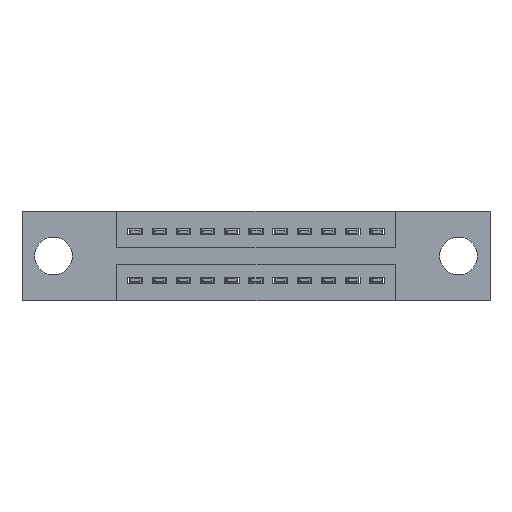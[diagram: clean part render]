
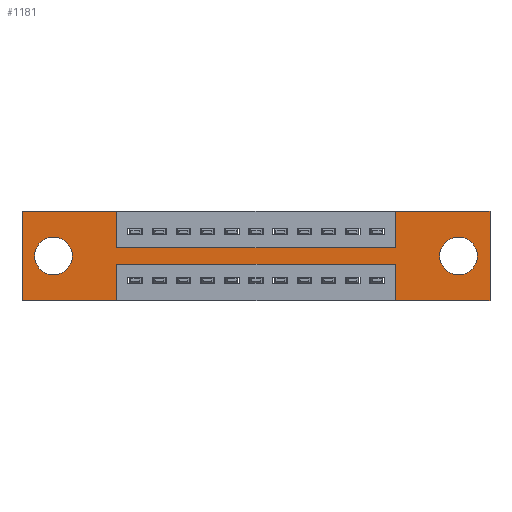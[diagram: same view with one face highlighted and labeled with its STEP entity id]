
A CAD part, front view. The second image highlights one B-rep face of the part: STEP entity #1181.
In plain terms, the highlighted planar face has unit normal (0, -1, 0).
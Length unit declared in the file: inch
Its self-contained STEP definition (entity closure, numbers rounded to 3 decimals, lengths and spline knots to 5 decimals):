
#24 = DIRECTION ( 'NONE',  ( 0., 0., -1. ) ) ;
#165 = EDGE_CURVE ( 'NONE', #11801, #4384, #6008, .T. ) ;
#247 = ORIENTED_EDGE ( 'NONE', *, *, #9492, .T. ) ;
#303 = DIRECTION ( 'NONE',  ( 0., 1., 0. ) ) ;
#377 = LINE ( 'NONE', #9774, #10524 ) ;
#446 = LINE ( 'NONE', #3167, #5166 ) ;
#485 = VECTOR ( 'NONE', #6870, 39.37008 ) ;
#511 = AXIS2_PLACEMENT_3D ( 'NONE', #3338, #11051, #2813 ) ;
#535 = CARTESIAN_POINT ( 'NONE',  ( 0.3925, 0., -0.15 ) ) ;
#619 = VECTOR ( 'NONE', #7497, 39.37008 ) ;
#682 = LINE ( 'NONE', #7815, #6014 ) ;
#769 = CIRCLE ( 'NONE', #1543, 0.078 ) ;
#784 = LINE ( 'NONE', #3765, #8325 ) ;
#936 = VECTOR ( 'NONE', #9405, 39.37008 ) ;
#1005 = VERTEX_POINT ( 'NONE', #3651 ) ;
#1015 = VERTEX_POINT ( 'NONE', #7721 ) ;
#1137 = ORIENTED_EDGE ( 'NONE', *, *, #5476, .F. ) ;
#1178 = CARTESIAN_POINT ( 'NONE',  ( 0.3925, 0., -0.22 ) ) ;
#1181 = ADVANCED_FACE ( 'NONE', ( #12139, #7328, #7035 ), #2074, .T. ) ;
#1235 = CARTESIAN_POINT ( 'NONE',  ( 1.805, 0., -0.185 ) ) ;
#1338 = DIRECTION ( 'NONE',  ( 0., 1., 0. ) ) ;
#1355 = EDGE_CURVE ( 'NONE', #3964, #2586, #2855, .T. ) ;
#1472 = ORIENTED_EDGE ( 'NONE', *, *, #9036, .F. ) ;
#1543 = AXIS2_PLACEMENT_3D ( 'NONE', #1235, #303, #24 ) ;
#1653 = VERTEX_POINT ( 'NONE', #2843 ) ;
#1767 = EDGE_CURVE ( 'NONE', #6382, #9145, #5819, .T. ) ;
#1768 = DIRECTION ( 'NONE',  ( 0., 0., -1. ) ) ;
#1961 = DIRECTION ( 'NONE',  ( 0., 0., -1. ) ) ;
#1983 = LINE ( 'NONE', #10677, #4322 ) ;
#2074 = PLANE ( 'NONE',  #511 ) ;
#2124 = CARTESIAN_POINT ( 'NONE',  ( 0.13, 0., -0.263 ) ) ;
#2142 = EDGE_CURVE ( 'NONE', #12505, #1005, #784, .T. ) ;
#2246 = CARTESIAN_POINT ( 'NONE',  ( 0., 0., 0. ) ) ;
#2266 = DIRECTION ( 'NONE',  ( -1., 0., 0. ) ) ;
#2586 = VERTEX_POINT ( 'NONE', #6044 ) ;
#2611 = CARTESIAN_POINT ( 'NONE',  ( 0.3925, 0., -0.15 ) ) ;
#2647 = EDGE_CURVE ( 'NONE', #2586, #3964, #769, .T. ) ;
#2775 = VECTOR ( 'NONE', #5669, 39.37008 ) ;
#2813 = DIRECTION ( 'NONE',  ( 0., 0., -1. ) ) ;
#2843 = CARTESIAN_POINT ( 'NONE',  ( 0.3925, 0., -0.37 ) ) ;
#2855 = CIRCLE ( 'NONE', #3879, 0.078 ) ;
#2893 = VECTOR ( 'NONE', #7533, 39.37008 ) ;
#3090 = EDGE_CURVE ( 'NONE', #9145, #7401, #446, .T. ) ;
#3167 = CARTESIAN_POINT ( 'NONE',  ( 0.3925, 0., -0.22 ) ) ;
#3282 = LINE ( 'NONE', #5580, #619 ) ;
#3287 = EDGE_CURVE ( 'NONE', #10883, #11947, #8447, .T. ) ;
#3338 = CARTESIAN_POINT ( 'NONE',  ( 0., 0., -0.37 ) ) ;
#3388 = ORIENTED_EDGE ( 'NONE', *, *, #3090, .F. ) ;
#3527 = EDGE_CURVE ( 'NONE', #1015, #12505, #1983, .T. ) ;
#3651 = CARTESIAN_POINT ( 'NONE',  ( 1.935, 0., -0.37 ) ) ;
#3652 = EDGE_CURVE ( 'NONE', #5473, #1015, #377, .T. ) ;
#3765 = CARTESIAN_POINT ( 'NONE',  ( 1.935, 0., 0. ) ) ;
#3879 = AXIS2_PLACEMENT_3D ( 'NONE', #6215, #10425, #11386 ) ;
#3964 = VERTEX_POINT ( 'NONE', #7365 ) ;
#4322 = VECTOR ( 'NONE', #10637, 39.37008 ) ;
#4384 = VERTEX_POINT ( 'NONE', #4719 ) ;
#4666 = CARTESIAN_POINT ( 'NONE',  ( 0., 0., -0.37 ) ) ;
#4672 = ORIENTED_EDGE ( 'NONE', *, *, #11517, .F. ) ;
#4719 = CARTESIAN_POINT ( 'NONE',  ( 0.3925, 0., 0. ) ) ;
#5069 = AXIS2_PLACEMENT_3D ( 'NONE', #12141, #12131, #12121 ) ;
#5166 = VECTOR ( 'NONE', #2266, 39.37008 ) ;
#5170 = ORIENTED_EDGE ( 'NONE', *, *, #11722, .F. ) ;
#5281 = CARTESIAN_POINT ( 'NONE',  ( 1.935, 0., 0. ) ) ;
#5473 = VERTEX_POINT ( 'NONE', #6232 ) ;
#5476 = EDGE_CURVE ( 'NONE', #9728, #11801, #9428, .T. ) ;
#5567 = ORIENTED_EDGE ( 'NONE', *, *, #2142, .F. ) ;
#5580 = CARTESIAN_POINT ( 'NONE',  ( 0.3925, 0., -0.37 ) ) ;
#5669 = DIRECTION ( 'NONE',  ( -1., 0., 0. ) ) ;
#5673 = CARTESIAN_POINT ( 'NONE',  ( 0.13, 0., -0.107 ) ) ;
#5819 = LINE ( 'NONE', #11579, #485 ) ;
#5951 = DIRECTION ( 'NONE',  ( 0., 0., 1. ) ) ;
#6008 = LINE ( 'NONE', #2246, #10837 ) ;
#6014 = VECTOR ( 'NONE', #1961, 39.37008 ) ;
#6044 = CARTESIAN_POINT ( 'NONE',  ( 1.805, 0., -0.107 ) ) ;
#6215 = CARTESIAN_POINT ( 'NONE',  ( 1.805, 0., -0.185 ) ) ;
#6232 = CARTESIAN_POINT ( 'NONE',  ( 1.5425, 0., -0.15 ) ) ;
#6259 = CARTESIAN_POINT ( 'NONE',  ( 0., 0., 0. ) ) ;
#6308 = EDGE_CURVE ( 'NONE', #6965, #5473, #6551, .T. ) ;
#6326 = EDGE_CURVE ( 'NONE', #7401, #1653, #3282, .T. ) ;
#6382 = VERTEX_POINT ( 'NONE', #11429 ) ;
#6551 = LINE ( 'NONE', #535, #936 ) ;
#6621 = EDGE_LOOP ( 'NONE', ( #9662, #7670 ) ) ;
#6629 = CARTESIAN_POINT ( 'NONE',  ( 0., 0., -0.37 ) ) ;
#6870 = DIRECTION ( 'NONE',  ( 0., 0., 1. ) ) ;
#6965 = VERTEX_POINT ( 'NONE', #2611 ) ;
#7035 = FACE_OUTER_BOUND ( 'NONE', #10829, .T. ) ;
#7263 = CARTESIAN_POINT ( 'NONE',  ( 0.13, 0., -0.185 ) ) ;
#7328 = FACE_BOUND ( 'NONE', #7961, .T. ) ;
#7365 = CARTESIAN_POINT ( 'NONE',  ( 1.805, 0., -0.263 ) ) ;
#7401 = VERTEX_POINT ( 'NONE', #1178 ) ;
#7497 = DIRECTION ( 'NONE',  ( 0., 0., -1. ) ) ;
#7533 = DIRECTION ( 'NONE',  ( -1., 0., 0. ) ) ;
#7668 = AXIS2_PLACEMENT_3D ( 'NONE', #7263, #1338, #8201 ) ;
#7670 = ORIENTED_EDGE ( 'NONE', *, *, #1355, .T. ) ;
#7721 = CARTESIAN_POINT ( 'NONE',  ( 1.5425, 0., 0. ) ) ;
#7815 = CARTESIAN_POINT ( 'NONE',  ( 0.3925, 0., 0. ) ) ;
#7961 = EDGE_LOOP ( 'NONE', ( #11447, #247 ) ) ;
#7978 = LINE ( 'NONE', #4666, #2775 ) ;
#8201 = DIRECTION ( 'NONE',  ( 0., 0., 1. ) ) ;
#8292 = ORIENTED_EDGE ( 'NONE', *, *, #1767, .F. ) ;
#8325 = VECTOR ( 'NONE', #1768, 39.37008 ) ;
#8447 = CIRCLE ( 'NONE', #5069, 0.078 ) ;
#8620 = ORIENTED_EDGE ( 'NONE', *, *, #3527, .F. ) ;
#8673 = CARTESIAN_POINT ( 'NONE',  ( 1.5425, 0., -0.22 ) ) ;
#8693 = ORIENTED_EDGE ( 'NONE', *, *, #6326, .F. ) ;
#8793 = VECTOR ( 'NONE', #5951, 39.37008 ) ;
#8820 = CARTESIAN_POINT ( 'NONE',  ( 0., 0., 0. ) ) ;
#9036 = EDGE_CURVE ( 'NONE', #1653, #9728, #7978, .T. ) ;
#9145 = VERTEX_POINT ( 'NONE', #8673 ) ;
#9217 = ORIENTED_EDGE ( 'NONE', *, *, #6308, .F. ) ;
#9405 = DIRECTION ( 'NONE',  ( 1., 0., 0. ) ) ;
#9428 = LINE ( 'NONE', #6259, #8793 ) ;
#9492 = EDGE_CURVE ( 'NONE', #11947, #10883, #11763, .T. ) ;
#9516 = ORIENTED_EDGE ( 'NONE', *, *, #165, .F. ) ;
#9662 = ORIENTED_EDGE ( 'NONE', *, *, #2647, .T. ) ;
#9722 = DIRECTION ( 'NONE',  ( 0., 0., 1. ) ) ;
#9727 = DIRECTION ( 'NONE',  ( 1., 0., 0. ) ) ;
#9728 = VERTEX_POINT ( 'NONE', #6629 ) ;
#9774 = CARTESIAN_POINT ( 'NONE',  ( 1.5425, 0., 0. ) ) ;
#10102 = ORIENTED_EDGE ( 'NONE', *, *, #3652, .F. ) ;
#10422 = CARTESIAN_POINT ( 'NONE',  ( 0., 0., -0.37 ) ) ;
#10425 = DIRECTION ( 'NONE',  ( 0., 1., 0. ) ) ;
#10524 = VECTOR ( 'NONE', #9722, 39.37008 ) ;
#10637 = DIRECTION ( 'NONE',  ( 1., 0., 0. ) ) ;
#10677 = CARTESIAN_POINT ( 'NONE',  ( 0., 0., 0. ) ) ;
#10682 = LINE ( 'NONE', #10422, #2893 ) ;
#10829 = EDGE_LOOP ( 'NONE', ( #8693, #3388, #8292, #4672, #5567, #8620, #10102, #9217, #5170, #9516, #1137, #1472 ) ) ;
#10837 = VECTOR ( 'NONE', #9727, 39.37008 ) ;
#10883 = VERTEX_POINT ( 'NONE', #5673 ) ;
#11051 = DIRECTION ( 'NONE',  ( 0., -1., 0. ) ) ;
#11386 = DIRECTION ( 'NONE',  ( 0., 0., -1. ) ) ;
#11429 = CARTESIAN_POINT ( 'NONE',  ( 1.5425, 0., -0.37 ) ) ;
#11447 = ORIENTED_EDGE ( 'NONE', *, *, #3287, .T. ) ;
#11517 = EDGE_CURVE ( 'NONE', #1005, #6382, #10682, .T. ) ;
#11579 = CARTESIAN_POINT ( 'NONE',  ( 1.5425, 0., -0.37 ) ) ;
#11722 = EDGE_CURVE ( 'NONE', #4384, #6965, #682, .T. ) ;
#11763 = CIRCLE ( 'NONE', #7668, 0.078 ) ;
#11801 = VERTEX_POINT ( 'NONE', #8820 ) ;
#11947 = VERTEX_POINT ( 'NONE', #2124 ) ;
#12121 = DIRECTION ( 'NONE',  ( 0., 0., 1. ) ) ;
#12131 = DIRECTION ( 'NONE',  ( 0., 1., 0. ) ) ;
#12139 = FACE_BOUND ( 'NONE', #6621, .T. ) ;
#12141 = CARTESIAN_POINT ( 'NONE',  ( 0.13, 0., -0.185 ) ) ;
#12505 = VERTEX_POINT ( 'NONE', #5281 ) ;
